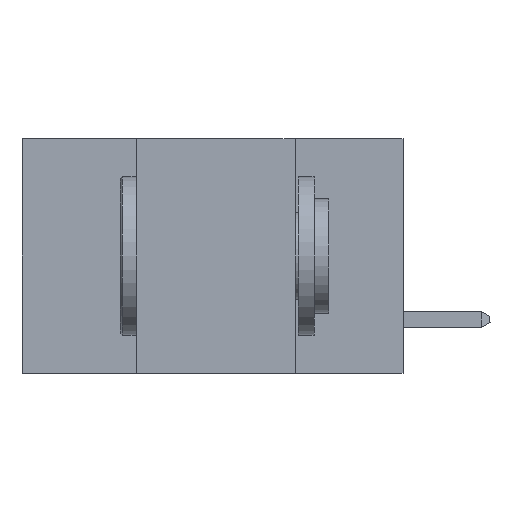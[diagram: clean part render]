
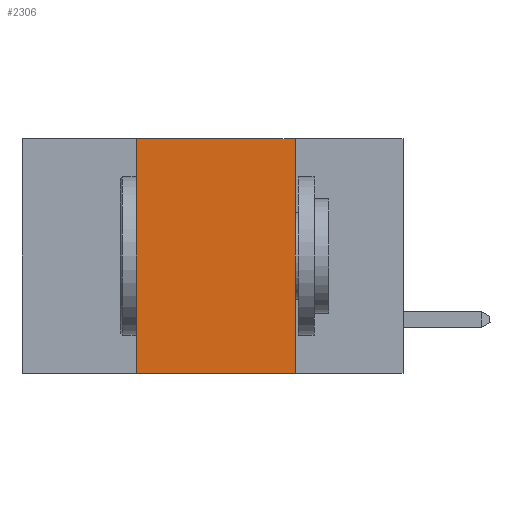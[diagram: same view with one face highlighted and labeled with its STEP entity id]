
A CAD part, left-side view. The second image highlights one B-rep face of the part: STEP entity #2306.
In plain terms, the highlighted planar face has unit normal (-1, 0, 0).
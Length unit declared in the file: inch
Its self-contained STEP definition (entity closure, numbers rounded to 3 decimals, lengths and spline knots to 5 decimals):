
#26 = DIRECTION ( 'NONE',  ( 0., 0., 1. ) ) ;
#895 = CARTESIAN_POINT ( 'NONE',  ( 0., 0.17, 0. ) ) ;
#1023 = DIRECTION ( 'NONE',  ( 0., -1., 0. ) ) ;
#1246 = CARTESIAN_POINT ( 'NONE',  ( 0., 0.17, 0. ) ) ;
#2306 = ADVANCED_FACE ( 'NONE', ( #14774 ), #19001, .F. ) ;
#2570 = VERTEX_POINT ( 'NONE', #14307 ) ;
#4048 = DIRECTION ( 'NONE',  ( 0., -1., 0. ) ) ;
#4228 = LINE ( 'NONE', #6091, #11301 ) ;
#4374 = VECTOR ( 'NONE', #4048, 39.37008 ) ;
#5122 = VECTOR ( 'NONE', #1023, 39.37008 ) ;
#5395 = DIRECTION ( 'NONE',  ( 1., 0., 0. ) ) ;
#5580 = LINE ( 'NONE', #19158, #5122 ) ;
#6091 = CARTESIAN_POINT ( 'NONE',  ( 0., 0.42, 0. ) ) ;
#7019 = DIRECTION ( 'NONE',  ( 0., 0., -1. ) ) ;
#8473 = EDGE_CURVE ( 'NONE', #12783, #9091, #5580, .T. ) ;
#8556 = CARTESIAN_POINT ( 'NONE',  ( 0., 0.6, 0. ) ) ;
#8854 = LINE ( 'NONE', #11431, #4374 ) ;
#9091 = VERTEX_POINT ( 'NONE', #1246 ) ;
#9139 = EDGE_CURVE ( 'NONE', #2570, #11034, #8854, .T. ) ;
#10537 = EDGE_LOOP ( 'NONE', ( #12081, #16158, #12725, #15356 ) ) ;
#11034 = VERTEX_POINT ( 'NONE', #13246 ) ;
#11301 = VECTOR ( 'NONE', #26, 39.37008 ) ;
#11431 = CARTESIAN_POINT ( 'NONE',  ( 0., 0.6, -0.37 ) ) ;
#12081 = ORIENTED_EDGE ( 'NONE', *, *, #18415, .F. ) ;
#12725 = ORIENTED_EDGE ( 'NONE', *, *, #15497, .F. ) ;
#12783 = VERTEX_POINT ( 'NONE', #16259 ) ;
#13246 = CARTESIAN_POINT ( 'NONE',  ( 0., 0.17, -0.37 ) ) ;
#14307 = CARTESIAN_POINT ( 'NONE',  ( 0., 0.42, -0.37 ) ) ;
#14774 = FACE_OUTER_BOUND ( 'NONE', #10537, .T. ) ;
#15078 = VECTOR ( 'NONE', #7019, 39.37008 ) ;
#15356 = ORIENTED_EDGE ( 'NONE', *, *, #9139, .T. ) ;
#15497 = EDGE_CURVE ( 'NONE', #2570, #12783, #4228, .T. ) ;
#16140 = AXIS2_PLACEMENT_3D ( 'NONE', #8556, #5395, #17433 ) ;
#16158 = ORIENTED_EDGE ( 'NONE', *, *, #8473, .F. ) ;
#16259 = CARTESIAN_POINT ( 'NONE',  ( 0., 0.42, 0. ) ) ;
#17433 = DIRECTION ( 'NONE',  ( 0., 0., -1. ) ) ;
#17846 = LINE ( 'NONE', #895, #15078 ) ;
#18415 = EDGE_CURVE ( 'NONE', #9091, #11034, #17846, .T. ) ;
#19001 = PLANE ( 'NONE',  #16140 ) ;
#19158 = CARTESIAN_POINT ( 'NONE',  ( 0., 0.6, 0. ) ) ;
